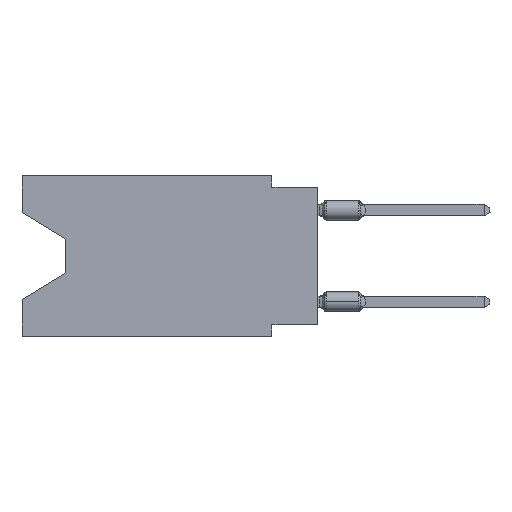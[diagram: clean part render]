
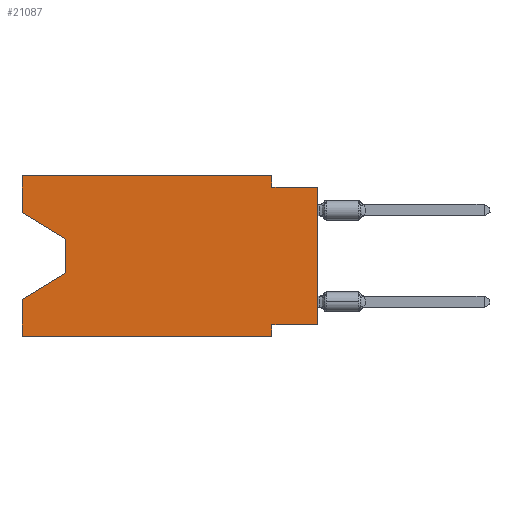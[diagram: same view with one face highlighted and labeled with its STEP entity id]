
A CAD part, left-side view. The second image highlights one B-rep face of the part: STEP entity #21087.
In plain terms, the highlighted planar face has unit normal (-1, 0, 0).
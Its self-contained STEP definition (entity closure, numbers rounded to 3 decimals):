
#787 = EDGE_CURVE ( 'NONE', #32557, #7060, #8504, .T. ) ;
#855 = ORIENTED_EDGE ( 'NONE', *, *, #20014, .F. ) ;
#1556 = DIRECTION ( 'NONE',  ( 0., 0., 1. ) ) ;
#1799 = VECTOR ( 'NONE', #53435, 1000. ) ;
#2445 = PLANE ( 'NONE',  #57153 ) ;
#2469 = LINE ( 'NONE', #11053, #51669 ) ;
#2582 = LINE ( 'NONE', #37669, #29857 ) ;
#2711 = CARTESIAN_POINT ( 'NONE',  ( 0., 0., 0. ) ) ;
#2763 = DIRECTION ( 'NONE',  ( 0., 1., 0. ) ) ;
#3520 = ORIENTED_EDGE ( 'NONE', *, *, #44281, .F. ) ;
#3775 = CARTESIAN_POINT ( 'NONE',  ( 0., 16.383, 0. ) ) ;
#4060 = LINE ( 'NONE', #48899, #37448 ) ;
#5694 = CARTESIAN_POINT ( 'NONE',  ( 0., 2.54, -8.89 ) ) ;
#6200 = CARTESIAN_POINT ( 'NONE',  ( 0., 2.54, -0.635 ) ) ;
#6365 = VECTOR ( 'NONE', #55582, 1000. ) ;
#6470 = VECTOR ( 'NONE', #2763, 1000. ) ;
#7051 = VERTEX_POINT ( 'NONE', #41961 ) ;
#7060 = VERTEX_POINT ( 'NONE', #5694 ) ;
#8504 = LINE ( 'NONE', #58100, #14720 ) ;
#9987 = EDGE_CURVE ( 'NONE', #32144, #7051, #49205, .T. ) ;
#11053 = CARTESIAN_POINT ( 'NONE',  ( 0., 13.97, -3.505 ) ) ;
#13225 = DIRECTION ( 'NONE',  ( 0., -1., 0. ) ) ;
#13746 = VECTOR ( 'NONE', #17613, 1000. ) ;
#14140 = CARTESIAN_POINT ( 'NONE',  ( 0., 13.97, -3.505 ) ) ;
#14720 = VECTOR ( 'NONE', #13225, 1000. ) ;
#15555 = VERTEX_POINT ( 'NONE', #14140 ) ;
#17052 = DIRECTION ( 'NONE',  ( 0., 0., 1. ) ) ;
#17382 = VERTEX_POINT ( 'NONE', #20304 ) ;
#17613 = DIRECTION ( 'NONE',  ( 0., 0., -1. ) ) ;
#18641 = CARTESIAN_POINT ( 'NONE',  ( 0., 0., -0.635 ) ) ;
#19238 = LINE ( 'NONE', #37221, #45737 ) ;
#19973 = DIRECTION ( 'NONE',  ( 0., -0.855, -0.519 ) ) ;
#20014 = EDGE_CURVE ( 'NONE', #36515, #30308, #40449, .T. ) ;
#20133 = CARTESIAN_POINT ( 'NONE',  ( 0., 16.383, 0. ) ) ;
#20304 = CARTESIAN_POINT ( 'NONE',  ( 0., 2.54, 0. ) ) ;
#20383 = EDGE_CURVE ( 'NONE', #17382, #36515, #40880, .T. ) ;
#20705 = CARTESIAN_POINT ( 'NONE',  ( 0., 13.97, -5.385 ) ) ;
#21087 = ADVANCED_FACE ( 'NONE', ( #30151 ), #2445, .F. ) ;
#21796 = CARTESIAN_POINT ( 'NONE',  ( 0., 2.54, -8.255 ) ) ;
#22386 = CARTESIAN_POINT ( 'NONE',  ( 0., 16.383, -8.89 ) ) ;
#23109 = VECTOR ( 'NONE', #1556, 1000. ) ;
#23287 = ORIENTED_EDGE ( 'NONE', *, *, #9987, .F. ) ;
#23596 = ORIENTED_EDGE ( 'NONE', *, *, #787, .T. ) ;
#26542 = VERTEX_POINT ( 'NONE', #42486 ) ;
#27621 = DIRECTION ( 'NONE',  ( 0., 0., 1. ) ) ;
#29554 = LINE ( 'NONE', #20705, #6365 ) ;
#29857 = VECTOR ( 'NONE', #19973, 1000. ) ;
#30151 = FACE_OUTER_BOUND ( 'NONE', #50823, .T. ) ;
#30308 = VERTEX_POINT ( 'NONE', #18641 ) ;
#31013 = DIRECTION ( 'NONE',  ( 0., -1., 0. ) ) ;
#31544 = CARTESIAN_POINT ( 'NONE',  ( 0., 16.383, 0. ) ) ;
#31549 = ORIENTED_EDGE ( 'NONE', *, *, #20383, .F. ) ;
#32144 = VERTEX_POINT ( 'NONE', #57888 ) ;
#32415 = VERTEX_POINT ( 'NONE', #48346 ) ;
#32557 = VERTEX_POINT ( 'NONE', #22386 ) ;
#33577 = ORIENTED_EDGE ( 'NONE', *, *, #43453, .F. ) ;
#34579 = DIRECTION ( 'NONE',  ( 0., 0., -1. ) ) ;
#34772 = ORIENTED_EDGE ( 'NONE', *, *, #50537, .T. ) ;
#36515 = VERTEX_POINT ( 'NONE', #6200 ) ;
#36809 = VERTEX_POINT ( 'NONE', #21796 ) ;
#37221 = CARTESIAN_POINT ( 'NONE',  ( 0., 2.54, -8.89 ) ) ;
#37448 = VECTOR ( 'NONE', #27621, 1000. ) ;
#37669 = CARTESIAN_POINT ( 'NONE',  ( 0., 16.383, -2.038 ) ) ;
#38869 = VECTOR ( 'NONE', #17052, 1000. ) ;
#39571 = CARTESIAN_POINT ( 'NONE',  ( 0., 0., -0.635 ) ) ;
#39887 = CARTESIAN_POINT ( 'NONE',  ( 0., 0., -8.255 ) ) ;
#40196 = EDGE_CURVE ( 'NONE', #15555, #26542, #2469, .T. ) ;
#40449 = LINE ( 'NONE', #39571, #51423 ) ;
#40719 = ORIENTED_EDGE ( 'NONE', *, *, #44803, .F. ) ;
#40880 = LINE ( 'NONE', #50040, #13746 ) ;
#41947 = LINE ( 'NONE', #2711, #23109 ) ;
#41961 = CARTESIAN_POINT ( 'NONE',  ( 0., 16.383, 0. ) ) ;
#42486 = CARTESIAN_POINT ( 'NONE',  ( 0., 13.97, -5.385 ) ) ;
#43423 = DIRECTION ( 'NONE',  ( 1., 0., 0. ) ) ;
#43453 = EDGE_CURVE ( 'NONE', #32557, #56709, #4060, .T. ) ;
#43734 = DIRECTION ( 'NONE',  ( 0., 0., -1. ) ) ;
#44115 = ORIENTED_EDGE ( 'NONE', *, *, #57594, .T. ) ;
#44281 = EDGE_CURVE ( 'NONE', #32415, #36809, #57346, .T. ) ;
#44726 = ORIENTED_EDGE ( 'NONE', *, *, #40196, .T. ) ;
#44803 = EDGE_CURVE ( 'NONE', #7051, #17382, #45702, .T. ) ;
#45702 = LINE ( 'NONE', #31544, #1799 ) ;
#45737 = VECTOR ( 'NONE', #46664, 1000. ) ;
#46664 = DIRECTION ( 'NONE',  ( 0., 0., -1. ) ) ;
#48346 = CARTESIAN_POINT ( 'NONE',  ( 0., 0., -8.255 ) ) ;
#48899 = CARTESIAN_POINT ( 'NONE',  ( 0., 16.383, 0. ) ) ;
#48966 = ORIENTED_EDGE ( 'NONE', *, *, #53178, .F. ) ;
#49205 = LINE ( 'NONE', #3775, #38869 ) ;
#50040 = CARTESIAN_POINT ( 'NONE',  ( 0., 2.54, 0. ) ) ;
#50537 = EDGE_CURVE ( 'NONE', #26542, #56709, #29554, .T. ) ;
#50823 = EDGE_LOOP ( 'NONE', ( #52716, #44726, #34772, #33577, #23596, #48966, #3520, #44115, #855, #31549, #40719, #23287 ) ) ;
#51423 = VECTOR ( 'NONE', #31013, 1000. ) ;
#51669 = VECTOR ( 'NONE', #43734, 1000. ) ;
#52610 = EDGE_CURVE ( 'NONE', #32144, #15555, #2582, .T. ) ;
#52716 = ORIENTED_EDGE ( 'NONE', *, *, #52610, .T. ) ;
#53178 = EDGE_CURVE ( 'NONE', #36809, #7060, #19238, .T. ) ;
#53435 = DIRECTION ( 'NONE',  ( 0., -1., 0. ) ) ;
#54097 = CARTESIAN_POINT ( 'NONE',  ( 0., 16.383, -6.852 ) ) ;
#55582 = DIRECTION ( 'NONE',  ( 0., 0.855, -0.519 ) ) ;
#56709 = VERTEX_POINT ( 'NONE', #54097 ) ;
#57153 = AXIS2_PLACEMENT_3D ( 'NONE', #20133, #43423, #34579 ) ;
#57346 = LINE ( 'NONE', #39887, #6470 ) ;
#57594 = EDGE_CURVE ( 'NONE', #32415, #30308, #41947, .T. ) ;
#57888 = CARTESIAN_POINT ( 'NONE',  ( 0., 16.383, -2.038 ) ) ;
#58100 = CARTESIAN_POINT ( 'NONE',  ( 0., 16.383, -8.89 ) ) ;
